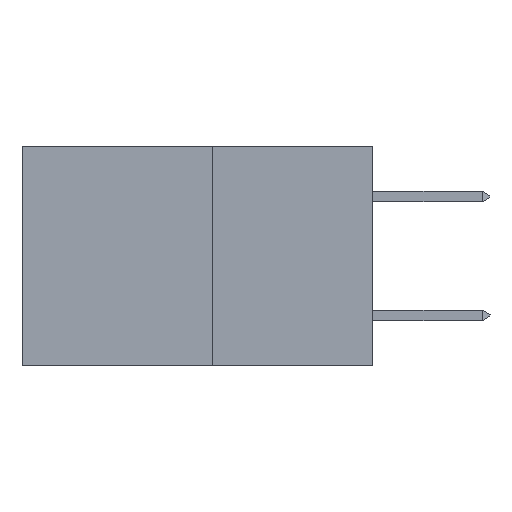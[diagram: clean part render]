
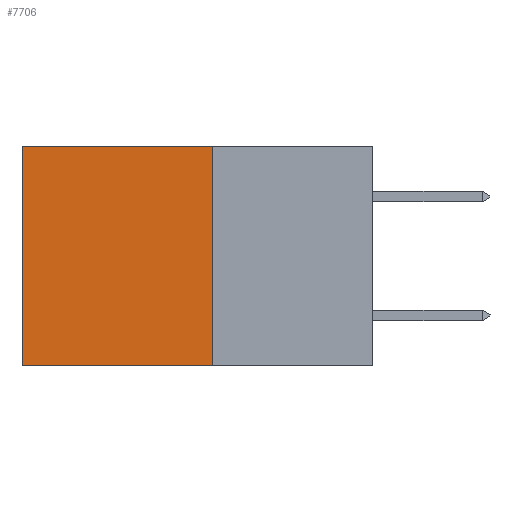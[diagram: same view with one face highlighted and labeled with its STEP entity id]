
A CAD part, left-side view. The second image highlights one B-rep face of the part: STEP entity #7706.
In plain terms, the highlighted planar face has unit normal (-1, 0, 0).
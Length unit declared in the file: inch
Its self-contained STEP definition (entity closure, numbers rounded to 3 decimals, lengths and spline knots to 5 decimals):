
#1114 = VERTEX_POINT ( 'NONE', #21191 ) ;
#1199 = CARTESIAN_POINT ( 'NONE',  ( 0.277, 0.59, -0.37 ) ) ;
#1615 = CARTESIAN_POINT ( 'NONE',  ( 0.277, 0.27, -0.37 ) ) ;
#1630 = CARTESIAN_POINT ( 'NONE',  ( 0.277, 0.27, -0.37 ) ) ;
#3298 = CARTESIAN_POINT ( 'NONE',  ( 0.277, 0.27, -0.37 ) ) ;
#3535 = VECTOR ( 'NONE', #5672, 39.37008 ) ;
#4009 = DIRECTION ( 'NONE',  ( 1., 0., 0. ) ) ;
#4933 = LINE ( 'NONE', #1615, #23790 ) ;
#5672 = DIRECTION ( 'NONE',  ( 0., 0., -1. ) ) ;
#6093 = AXIS2_PLACEMENT_3D ( 'NONE', #1630, #4009, #20614 ) ;
#6146 = CARTESIAN_POINT ( 'NONE',  ( 0.277, 0.59, -0.37 ) ) ;
#6457 = ORIENTED_EDGE ( 'NONE', *, *, #7498, .F. ) ;
#6539 = ORIENTED_EDGE ( 'NONE', *, *, #25989, .T. ) ;
#7094 = EDGE_LOOP ( 'NONE', ( #25625, #26008, #6457, #6539 ) ) ;
#7498 = EDGE_CURVE ( 'NONE', #22962, #8047, #27153, .T. ) ;
#7628 = VERTEX_POINT ( 'NONE', #1199 ) ;
#7706 = ADVANCED_FACE ( 'NONE', ( #27528 ), #15821, .F. ) ;
#8047 = VERTEX_POINT ( 'NONE', #23931 ) ;
#8262 = VECTOR ( 'NONE', #25051, 39.37008 ) ;
#15811 = DIRECTION ( 'NONE',  ( 0., 1., 0. ) ) ;
#15821 = PLANE ( 'NONE',  #6093 ) ;
#16197 = EDGE_CURVE ( 'NONE', #8047, #7628, #4933, .T. ) ;
#16753 = EDGE_CURVE ( 'NONE', #1114, #7628, #27784, .T. ) ;
#17877 = CARTESIAN_POINT ( 'NONE',  ( 0.277, 0.27, 0. ) ) ;
#20614 = DIRECTION ( 'NONE',  ( 0., 0., -1. ) ) ;
#21191 = CARTESIAN_POINT ( 'NONE',  ( 0.277, 0.59, 0. ) ) ;
#22962 = VERTEX_POINT ( 'NONE', #17877 ) ;
#23308 = DIRECTION ( 'NONE',  ( 0., 1., 0. ) ) ;
#23790 = VECTOR ( 'NONE', #15811, 39.37008 ) ;
#23931 = CARTESIAN_POINT ( 'NONE',  ( 0.277, 0.27, -0.37 ) ) ;
#25051 = DIRECTION ( 'NONE',  ( 0., 0., -1. ) ) ;
#25405 = LINE ( 'NONE', #30318, #30231 ) ;
#25625 = ORIENTED_EDGE ( 'NONE', *, *, #16753, .T. ) ;
#25989 = EDGE_CURVE ( 'NONE', #22962, #1114, #25405, .T. ) ;
#26008 = ORIENTED_EDGE ( 'NONE', *, *, #16197, .F. ) ;
#27153 = LINE ( 'NONE', #3298, #3535 ) ;
#27528 = FACE_OUTER_BOUND ( 'NONE', #7094, .T. ) ;
#27784 = LINE ( 'NONE', #6146, #8262 ) ;
#30231 = VECTOR ( 'NONE', #23308, 39.37008 ) ;
#30318 = CARTESIAN_POINT ( 'NONE',  ( 0.277, 0.27, 0. ) ) ;
